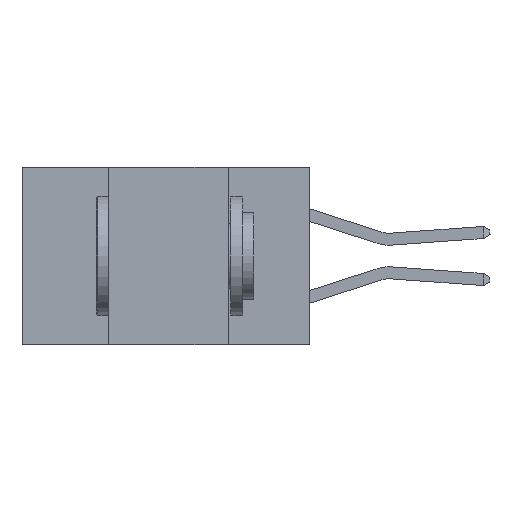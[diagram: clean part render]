
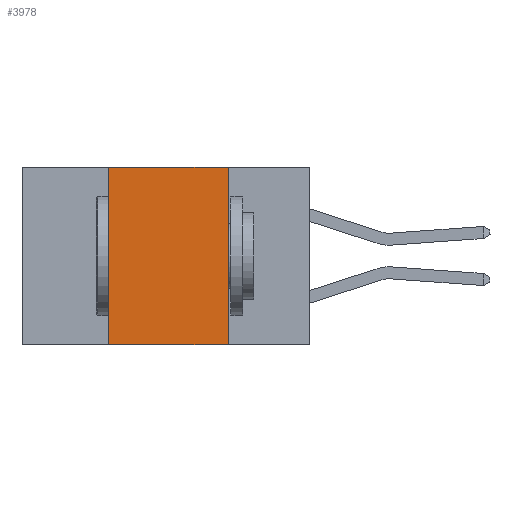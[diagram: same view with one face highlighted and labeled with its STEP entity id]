
A CAD part, left-side view. The second image highlights one B-rep face of the part: STEP entity #3978.
In plain terms, the highlighted planar face has unit normal (-1, 0, 0).
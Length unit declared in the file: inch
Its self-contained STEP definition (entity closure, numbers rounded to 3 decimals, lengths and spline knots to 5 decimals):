
#1072 = VERTEX_POINT ( 'NONE', #22171 ) ;
#1513 = ORIENTED_EDGE ( 'NONE', *, *, #5400, .F. ) ;
#1968 = VECTOR ( 'NONE', #19086, 39.37008 ) ;
#3399 = DIRECTION ( 'NONE',  ( 1., 0., 0. ) ) ;
#3978 = ADVANCED_FACE ( 'NONE', ( #17491 ), #19218, .F. ) ;
#4487 = ORIENTED_EDGE ( 'NONE', *, *, #10309, .F. ) ;
#5012 = LINE ( 'NONE', #12042, #1968 ) ;
#5400 = EDGE_CURVE ( 'NONE', #1072, #14065, #5012, .T. ) ;
#5829 = CARTESIAN_POINT ( 'NONE',  ( 0., 0.17, -0.37 ) ) ;
#5860 = CARTESIAN_POINT ( 'NONE',  ( 0., 0.6, 0. ) ) ;
#6787 = CARTESIAN_POINT ( 'NONE',  ( 0., 0.6, -0.37 ) ) ;
#7007 = LINE ( 'NONE', #6787, #19645 ) ;
#7184 = EDGE_CURVE ( 'NONE', #1072, #15811, #7007, .T. ) ;
#8308 = VECTOR ( 'NONE', #20893, 39.37008 ) ;
#8496 = DIRECTION ( 'NONE',  ( 0., 0., -1. ) ) ;
#9199 = LINE ( 'NONE', #5860, #8308 ) ;
#10194 = CARTESIAN_POINT ( 'NONE',  ( 0., 0.17, -0.37 ) ) ;
#10309 = EDGE_CURVE ( 'NONE', #17784, #15811, #17219, .T. ) ;
#12042 = CARTESIAN_POINT ( 'NONE',  ( 0., 0.42, -0.37 ) ) ;
#12079 = CARTESIAN_POINT ( 'NONE',  ( 0., 0.6, 0. ) ) ;
#12307 = ORIENTED_EDGE ( 'NONE', *, *, #22138, .F. ) ;
#12500 = AXIS2_PLACEMENT_3D ( 'NONE', #12079, #3399, #8496 ) ;
#13495 = VECTOR ( 'NONE', #20671, 39.37008 ) ;
#14065 = VERTEX_POINT ( 'NONE', #21095 ) ;
#15429 = ORIENTED_EDGE ( 'NONE', *, *, #7184, .T. ) ;
#15784 = EDGE_LOOP ( 'NONE', ( #4487, #12307, #1513, #15429 ) ) ;
#15811 = VERTEX_POINT ( 'NONE', #5829 ) ;
#17219 = LINE ( 'NONE', #10194, #13495 ) ;
#17371 = DIRECTION ( 'NONE',  ( 0., -1., 0. ) ) ;
#17491 = FACE_OUTER_BOUND ( 'NONE', #15784, .T. ) ;
#17784 = VERTEX_POINT ( 'NONE', #22196 ) ;
#19086 = DIRECTION ( 'NONE',  ( 0., 0., 1. ) ) ;
#19218 = PLANE ( 'NONE',  #12500 ) ;
#19645 = VECTOR ( 'NONE', #17371, 39.37008 ) ;
#20671 = DIRECTION ( 'NONE',  ( 0., 0., -1. ) ) ;
#20893 = DIRECTION ( 'NONE',  ( 0., -1., 0. ) ) ;
#21095 = CARTESIAN_POINT ( 'NONE',  ( 0., 0.42, 0. ) ) ;
#22138 = EDGE_CURVE ( 'NONE', #14065, #17784, #9199, .T. ) ;
#22171 = CARTESIAN_POINT ( 'NONE',  ( 0., 0.42, -0.37 ) ) ;
#22196 = CARTESIAN_POINT ( 'NONE',  ( 0., 0.17, 0. ) ) ;
